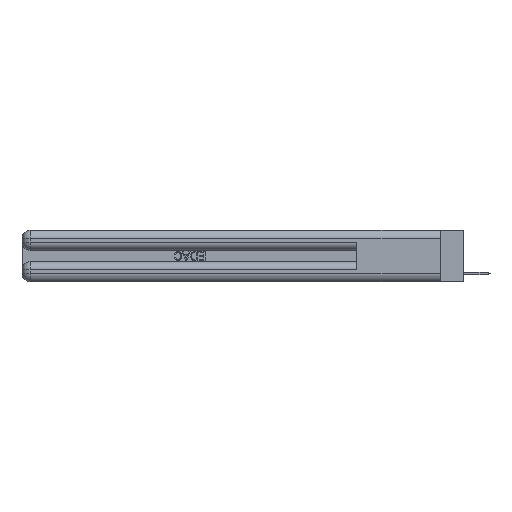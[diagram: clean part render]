
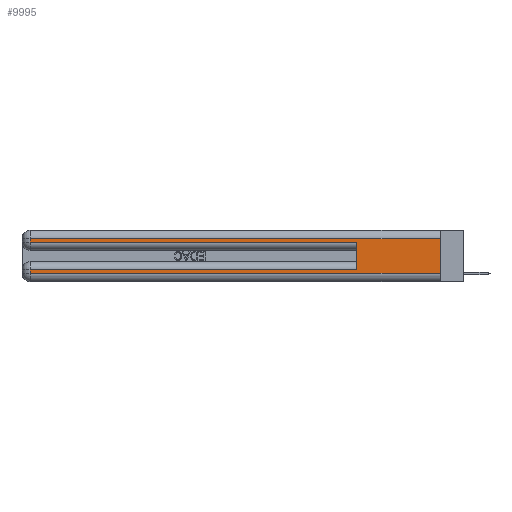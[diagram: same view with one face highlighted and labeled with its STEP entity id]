
A CAD part, left-side view. The second image highlights one B-rep face of the part: STEP entity #9995.
In plain terms, the highlighted planar face has unit normal (-1, 0, 0).
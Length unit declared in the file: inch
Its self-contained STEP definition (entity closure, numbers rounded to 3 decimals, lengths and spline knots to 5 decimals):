
#507 = VECTOR ( 'NONE', #26002, 39.37008 ) ;
#722 = VERTEX_POINT ( 'NONE', #1651 ) ;
#807 = VECTOR ( 'NONE', #19484, 39.37008 ) ;
#1155 = VERTEX_POINT ( 'NONE', #4450 ) ;
#1217 = CARTESIAN_POINT ( 'NONE',  ( 0., 0., 0.285 ) ) ;
#1543 = CARTESIAN_POINT ( 'NONE',  ( 0., 2.94, 0.06 ) ) ;
#1651 = CARTESIAN_POINT ( 'NONE',  ( 0., 0.6, 0.085 ) ) ;
#1934 = ORIENTED_EDGE ( 'NONE', *, *, #24790, .T. ) ;
#2334 = ORIENTED_EDGE ( 'NONE', *, *, #28403, .T. ) ;
#2359 = LINE ( 'NONE', #25657, #25935 ) ;
#2500 = EDGE_CURVE ( 'NONE', #3116, #28101, #18361, .T. ) ;
#2566 = CARTESIAN_POINT ( 'NONE',  ( 0., 0., 0.06 ) ) ;
#3116 = VERTEX_POINT ( 'NONE', #27549 ) ;
#3782 = CARTESIAN_POINT ( 'NONE',  ( 0., 2.94, 0.37 ) ) ;
#4450 = CARTESIAN_POINT ( 'NONE',  ( 0., 2.94, 0.31 ) ) ;
#4555 = CARTESIAN_POINT ( 'NONE',  ( 0., 0., 0.31 ) ) ;
#4646 = DIRECTION ( 'NONE',  ( 0., 1., 0. ) ) ;
#4822 = DIRECTION ( 'NONE',  ( 0., 0., -1. ) ) ;
#5029 = ORIENTED_EDGE ( 'NONE', *, *, #2500, .F. ) ;
#5561 = ORIENTED_EDGE ( 'NONE', *, *, #14023, .T. ) ;
#5892 = LINE ( 'NONE', #4555, #25554 ) ;
#7854 = VERTEX_POINT ( 'NONE', #27891 ) ;
#7908 = LINE ( 'NONE', #11797, #23999 ) ;
#7960 = FACE_OUTER_BOUND ( 'NONE', #27575, .T. ) ;
#9087 = VERTEX_POINT ( 'NONE', #17026 ) ;
#9538 = CARTESIAN_POINT ( 'NONE',  ( 0., 0., 0.37 ) ) ;
#9995 = ADVANCED_FACE ( 'NONE', ( #7960 ), #18519, .F. ) ;
#10120 = ORIENTED_EDGE ( 'NONE', *, *, #16297, .F. ) ;
#11797 = CARTESIAN_POINT ( 'NONE',  ( 0., 0.6, 0.145 ) ) ;
#12064 = CARTESIAN_POINT ( 'NONE',  ( 0., 0., 0.06 ) ) ;
#12271 = VECTOR ( 'NONE', #24599, 39.37008 ) ;
#13034 = CARTESIAN_POINT ( 'NONE',  ( 0., 2.94, 0.37 ) ) ;
#13749 = EDGE_CURVE ( 'NONE', #722, #21204, #2359, .T. ) ;
#13968 = VECTOR ( 'NONE', #24458, 39.37008 ) ;
#14023 = EDGE_CURVE ( 'NONE', #24167, #28101, #15232, .T. ) ;
#14263 = EDGE_CURVE ( 'NONE', #3116, #1155, #5892, .T. ) ;
#15232 = LINE ( 'NONE', #2566, #16676 ) ;
#15491 = LINE ( 'NONE', #13034, #12271 ) ;
#16120 = LINE ( 'NONE', #3782, #13968 ) ;
#16297 = EDGE_CURVE ( 'NONE', #722, #9087, #7908, .T. ) ;
#16676 = VECTOR ( 'NONE', #27757, 39.37008 ) ;
#17026 = CARTESIAN_POINT ( 'NONE',  ( 0., 0.6, 0.285 ) ) ;
#17120 = ORIENTED_EDGE ( 'NONE', *, *, #13749, .T. ) ;
#18361 = LINE ( 'NONE', #21660, #507 ) ;
#18519 = PLANE ( 'NONE',  #21094 ) ;
#19484 = DIRECTION ( 'NONE',  ( 0., -1., 0. ) ) ;
#20681 = DIRECTION ( 'NONE',  ( 0., 1., 0. ) ) ;
#21094 = AXIS2_PLACEMENT_3D ( 'NONE', #9538, #25288, #4822 ) ;
#21204 = VERTEX_POINT ( 'NONE', #22874 ) ;
#21660 = CARTESIAN_POINT ( 'NONE',  ( 0., 0., 0.37 ) ) ;
#21954 = ORIENTED_EDGE ( 'NONE', *, *, #14263, .T. ) ;
#22874 = CARTESIAN_POINT ( 'NONE',  ( 0., 2.94, 0.085 ) ) ;
#23999 = VECTOR ( 'NONE', #25241, 39.37008 ) ;
#24167 = VERTEX_POINT ( 'NONE', #1543 ) ;
#24458 = DIRECTION ( 'NONE',  ( 0., 0., -1. ) ) ;
#24599 = DIRECTION ( 'NONE',  ( 0., 0., -1. ) ) ;
#24691 = LINE ( 'NONE', #1217, #807 ) ;
#24790 = EDGE_CURVE ( 'NONE', #7854, #9087, #24691, .T. ) ;
#24863 = EDGE_CURVE ( 'NONE', #21204, #24167, #16120, .T. ) ;
#25163 = ORIENTED_EDGE ( 'NONE', *, *, #24863, .T. ) ;
#25241 = DIRECTION ( 'NONE',  ( 0., 0., 1. ) ) ;
#25288 = DIRECTION ( 'NONE',  ( 1., 0., 0. ) ) ;
#25554 = VECTOR ( 'NONE', #4646, 39.37008 ) ;
#25657 = CARTESIAN_POINT ( 'NONE',  ( 0., 0., 0.085 ) ) ;
#25935 = VECTOR ( 'NONE', #20681, 39.37008 ) ;
#26002 = DIRECTION ( 'NONE',  ( 0., 0., -1. ) ) ;
#27549 = CARTESIAN_POINT ( 'NONE',  ( 0., 0., 0.31 ) ) ;
#27575 = EDGE_LOOP ( 'NONE', ( #5029, #21954, #2334, #1934, #10120, #17120, #25163, #5561 ) ) ;
#27757 = DIRECTION ( 'NONE',  ( 0., -1., 0. ) ) ;
#27891 = CARTESIAN_POINT ( 'NONE',  ( 0., 2.94, 0.285 ) ) ;
#28101 = VERTEX_POINT ( 'NONE', #12064 ) ;
#28403 = EDGE_CURVE ( 'NONE', #1155, #7854, #15491, .T. ) ;
